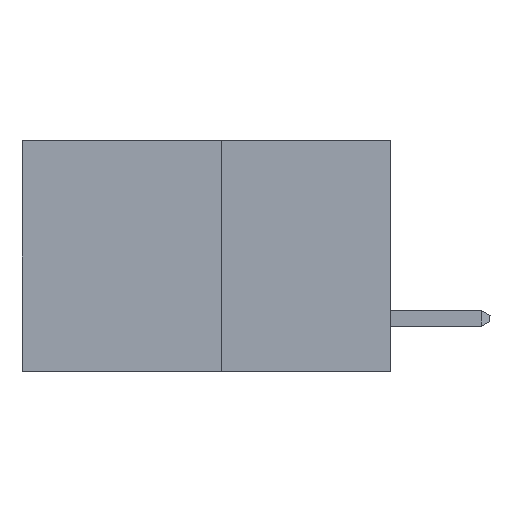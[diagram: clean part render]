
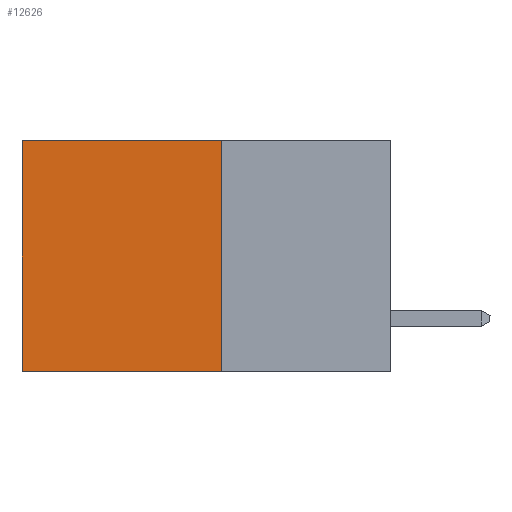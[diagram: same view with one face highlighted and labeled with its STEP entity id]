
A CAD part, left-side view. The second image highlights one B-rep face of the part: STEP entity #12626.
In plain terms, the highlighted planar face has unit normal (-1, 0, 0).
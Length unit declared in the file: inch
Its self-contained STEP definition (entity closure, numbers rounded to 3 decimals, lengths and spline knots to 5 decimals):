
#542 = FACE_OUTER_BOUND ( 'NONE', #4160, .T. ) ;
#1592 = AXIS2_PLACEMENT_3D ( 'NONE', #11860, #8575, #1773 ) ;
#1630 = LINE ( 'NONE', #8190, #10318 ) ;
#1773 = DIRECTION ( 'NONE',  ( 0., 0., -1. ) ) ;
#2695 = VERTEX_POINT ( 'NONE', #3987 ) ;
#3564 = EDGE_CURVE ( 'NONE', #2695, #6912, #9085, .T. ) ;
#3987 = CARTESIAN_POINT ( 'NONE',  ( 0.277, 0.27, -0.37 ) ) ;
#4045 = CARTESIAN_POINT ( 'NONE',  ( 0.277, 0.59, -0.37 ) ) ;
#4160 = EDGE_LOOP ( 'NONE', ( #10215, #8809, #8720, #14507 ) ) ;
#4868 = DIRECTION ( 'NONE',  ( 0., 1., 0. ) ) ;
#6912 = VERTEX_POINT ( 'NONE', #4045 ) ;
#7399 = PLANE ( 'NONE',  #1592 ) ;
#7679 = VERTEX_POINT ( 'NONE', #12043 ) ;
#7696 = CARTESIAN_POINT ( 'NONE',  ( 0.277, 0.59, -0.37 ) ) ;
#7758 = EDGE_CURVE ( 'NONE', #12226, #6912, #12883, .T. ) ;
#8190 = CARTESIAN_POINT ( 'NONE',  ( 0.277, 0.27, 0. ) ) ;
#8393 = VECTOR ( 'NONE', #9221, 39.37008 ) ;
#8575 = DIRECTION ( 'NONE',  ( 1., 0., 0. ) ) ;
#8720 = ORIENTED_EDGE ( 'NONE', *, *, #9145, .F. ) ;
#8809 = ORIENTED_EDGE ( 'NONE', *, *, #3564, .F. ) ;
#9085 = LINE ( 'NONE', #12804, #11674 ) ;
#9145 = EDGE_CURVE ( 'NONE', #7679, #2695, #11341, .T. ) ;
#9202 = EDGE_CURVE ( 'NONE', #7679, #12226, #1630, .T. ) ;
#9221 = DIRECTION ( 'NONE',  ( 0., 0., -1. ) ) ;
#9611 = VECTOR ( 'NONE', #13227, 39.37008 ) ;
#10215 = ORIENTED_EDGE ( 'NONE', *, *, #7758, .T. ) ;
#10318 = VECTOR ( 'NONE', #4868, 39.37008 ) ;
#11341 = LINE ( 'NONE', #13600, #8393 ) ;
#11674 = VECTOR ( 'NONE', #12605, 39.37008 ) ;
#11860 = CARTESIAN_POINT ( 'NONE',  ( 0.277, 0.27, -0.37 ) ) ;
#12043 = CARTESIAN_POINT ( 'NONE',  ( 0.277, 0.27, 0. ) ) ;
#12226 = VERTEX_POINT ( 'NONE', #14413 ) ;
#12605 = DIRECTION ( 'NONE',  ( 0., 1., 0. ) ) ;
#12626 = ADVANCED_FACE ( 'NONE', ( #542 ), #7399, .F. ) ;
#12804 = CARTESIAN_POINT ( 'NONE',  ( 0.277, 0.27, -0.37 ) ) ;
#12883 = LINE ( 'NONE', #7696, #9611 ) ;
#13227 = DIRECTION ( 'NONE',  ( 0., 0., -1. ) ) ;
#13600 = CARTESIAN_POINT ( 'NONE',  ( 0.277, 0.27, -0.37 ) ) ;
#14413 = CARTESIAN_POINT ( 'NONE',  ( 0.277, 0.59, 0. ) ) ;
#14507 = ORIENTED_EDGE ( 'NONE', *, *, #9202, .T. ) ;
